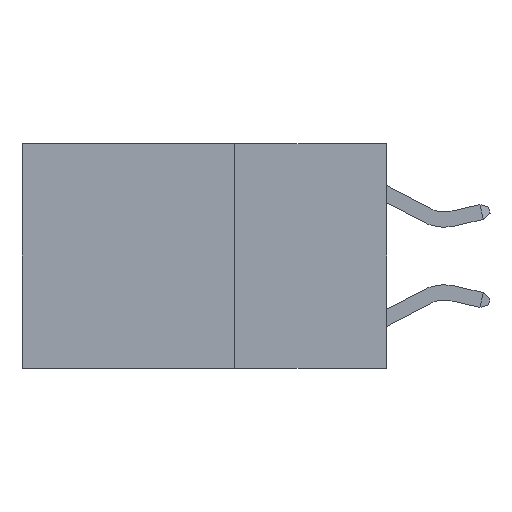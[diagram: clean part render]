
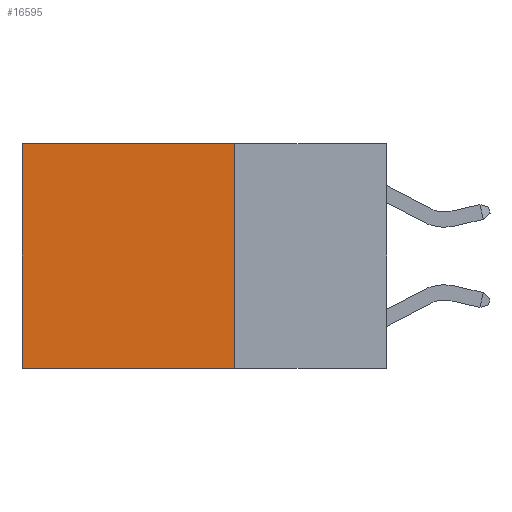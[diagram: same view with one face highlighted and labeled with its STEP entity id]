
A CAD part, left-side view. The second image highlights one B-rep face of the part: STEP entity #16595.
In plain terms, the highlighted planar face has unit normal (-1, 0, 0).
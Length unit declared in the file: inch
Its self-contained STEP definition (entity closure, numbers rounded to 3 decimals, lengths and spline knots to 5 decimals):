
#157 = CARTESIAN_POINT ( 'NONE',  ( 0.2625, 0.25, -0.37 ) ) ;
#229 = LINE ( 'NONE', #10403, #4083 ) ;
#706 = DIRECTION ( 'NONE',  ( 0., 0., -1. ) ) ;
#937 = EDGE_CURVE ( 'NONE', #10171, #5392, #13009, .T. ) ;
#1395 = DIRECTION ( 'NONE',  ( 0., 0., -1. ) ) ;
#3962 = VECTOR ( 'NONE', #7582, 39.37008 ) ;
#4083 = VECTOR ( 'NONE', #706, 39.37008 ) ;
#5392 = VERTEX_POINT ( 'NONE', #7460 ) ;
#7090 = EDGE_CURVE ( 'NONE', #11123, #5392, #19564, .T. ) ;
#7285 = ORIENTED_EDGE ( 'NONE', *, *, #18244, .T. ) ;
#7460 = CARTESIAN_POINT ( 'NONE',  ( 0.2625, 0.6, -0.37 ) ) ;
#7492 = EDGE_CURVE ( 'NONE', #19955, #10171, #229, .T. ) ;
#7582 = DIRECTION ( 'NONE',  ( 0., 1., 0. ) ) ;
#8343 = CARTESIAN_POINT ( 'NONE',  ( 0.2625, 0.25, 0. ) ) ;
#8666 = VECTOR ( 'NONE', #19117, 39.37008 ) ;
#9322 = DIRECTION ( 'NONE',  ( 0., 0., -1. ) ) ;
#10171 = VERTEX_POINT ( 'NONE', #157 ) ;
#10403 = CARTESIAN_POINT ( 'NONE',  ( 0.2625, 0.25, 0. ) ) ;
#10448 = VECTOR ( 'NONE', #1395, 39.37008 ) ;
#11123 = VERTEX_POINT ( 'NONE', #20152 ) ;
#11810 = ORIENTED_EDGE ( 'NONE', *, *, #7492, .F. ) ;
#12087 = ORIENTED_EDGE ( 'NONE', *, *, #937, .F. ) ;
#12624 = EDGE_LOOP ( 'NONE', ( #16438, #12087, #11810, #7285 ) ) ;
#13009 = LINE ( 'NONE', #14249, #8666 ) ;
#13561 = LINE ( 'NONE', #15652, #3962 ) ;
#14158 = CARTESIAN_POINT ( 'NONE',  ( 0.2625, 0.25, 0. ) ) ;
#14249 = CARTESIAN_POINT ( 'NONE',  ( 0.2625, 0.25, -0.37 ) ) ;
#14337 = CARTESIAN_POINT ( 'NONE',  ( 0.2625, 0.6, 0. ) ) ;
#15652 = CARTESIAN_POINT ( 'NONE',  ( 0.2625, 0.25, 0. ) ) ;
#16438 = ORIENTED_EDGE ( 'NONE', *, *, #7090, .T. ) ;
#16595 = ADVANCED_FACE ( 'NONE', ( #19680 ), #17412, .F. ) ;
#17412 = PLANE ( 'NONE',  #17560 ) ;
#17560 = AXIS2_PLACEMENT_3D ( 'NONE', #14158, #19017, #9322 ) ;
#18244 = EDGE_CURVE ( 'NONE', #19955, #11123, #13561, .T. ) ;
#19017 = DIRECTION ( 'NONE',  ( 1., 0., 0. ) ) ;
#19117 = DIRECTION ( 'NONE',  ( 0., 1., 0. ) ) ;
#19564 = LINE ( 'NONE', #14337, #10448 ) ;
#19680 = FACE_OUTER_BOUND ( 'NONE', #12624, .T. ) ;
#19955 = VERTEX_POINT ( 'NONE', #8343 ) ;
#20152 = CARTESIAN_POINT ( 'NONE',  ( 0.2625, 0.6, 0. ) ) ;
